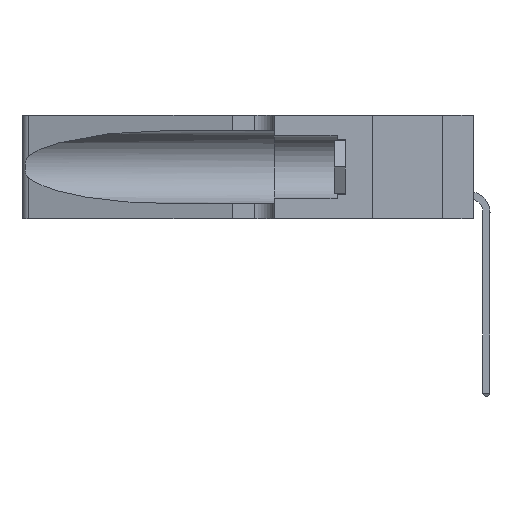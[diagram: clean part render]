
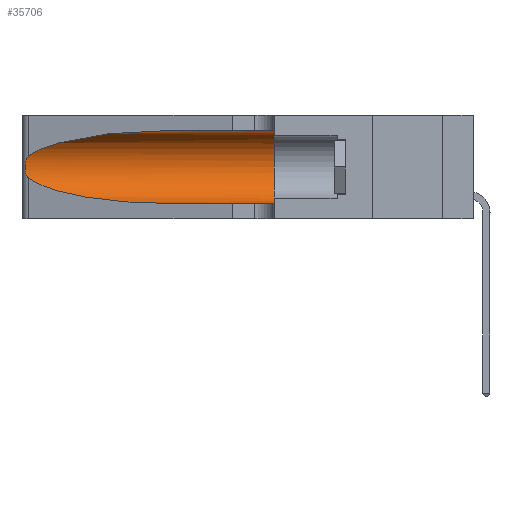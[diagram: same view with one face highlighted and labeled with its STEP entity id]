
A CAD part, left-side view. The second image highlights one B-rep face of the part: STEP entity #35706.
In plain terms, the highlighted cylindrical face has radius 3.308 mm (diameter 6.617 mm), a partial arc.
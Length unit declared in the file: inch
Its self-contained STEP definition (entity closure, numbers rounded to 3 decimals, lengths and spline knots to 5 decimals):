
#570 = CARTESIAN_POINT ( 'NONE',  ( 0.1305, 0.35, 0.05475 ) ) ;
#828 = EDGE_CURVE ( 'NONE', #36275, #28093, #7726, .T. ) ;
#1147 = CARTESIAN_POINT ( 'NONE',  ( 0.25487, 1.22718, 0.22369 ) ) ;
#1458 = CARTESIAN_POINT ( 'NONE',  ( 0.26075, 1.23896, 0.178 ) ) ;
#1589 = CARTESIAN_POINT ( 'NONE',  ( 0.25639, 1.23184, 0.21858 ) ) ;
#1686 = CARTESIAN_POINT ( 'NONE',  ( 0.1305, 0.72297, 0.31525 ) ) ;
#1888 = VERTEX_POINT ( 'NONE', #17448 ) ;
#1955 = CARTESIAN_POINT ( 'NONE',  ( 0.25487, 1.22718, 0.14631 ) ) ;
#2973 = DIRECTION ( 'NONE',  ( 0., -1., 0. ) ) ;
#3993 = CARTESIAN_POINT ( 'NONE',  ( 0.25555, 1.22994, 0.2215 ) ) ;
#4387 = CARTESIAN_POINT ( 'NONE',  ( 0.26017, 1.23833, 0.17102 ) ) ;
#5636 = EDGE_CURVE ( 'NONE', #1888, #11898, #5733, .T. ) ;
#5733 = CIRCLE ( 'NONE', #7338, 0.13025 ) ;
#6568 = CARTESIAN_POINT ( 'NONE',  ( 0.25487, 1.22718, 0.14631 ) ) ;
#7338 = AXIS2_PLACEMENT_3D ( 'NONE', #31438, #34355, #36896 ) ;
#7726 =( BOUNDED_CURVE ( )  B_SPLINE_CURVE ( 3, ( #1955, #13411, #25241, #36933 ),
 .UNSPECIFIED., .F., .T. ) 
 B_SPLINE_CURVE_WITH_KNOTS ( ( 4, 4 ),
 ( 3.44316, 4.71239 ),
 .UNSPECIFIED. ) 
 CURVE ( )  GEOMETRIC_REPRESENTATION_ITEM ( )  RATIONAL_B_SPLINE_CURVE ( ( 1., 0.87, 0.87, 1. ) ) 
 REPRESENTATION_ITEM ( '' )  );
#7829 = EDGE_LOOP ( 'NONE', ( #23922, #30203, #32178, #22317, #20930, #14837 ) ) ;
#7973 = CARTESIAN_POINT ( 'NONE',  ( 0.1305, 0.72297, 0.31525 ) ) ;
#8555 = VECTOR ( 'NONE', #23010, 39.37008 ) ;
#10827 = AXIS2_PLACEMENT_3D ( 'NONE', #21777, #24721, #27781 ) ;
#11898 = VERTEX_POINT ( 'NONE', #570 ) ;
#12617 = LINE ( 'NONE', #14281, #8555 ) ;
#13159 = CARTESIAN_POINT ( 'NONE',  ( 0.25639, 1.23186, 0.15144 ) ) ;
#13266 = CARTESIAN_POINT ( 'NONE',  ( 0.25487, 1.22718, 0.22369 ) ) ;
#13324 = EDGE_CURVE ( 'NONE', #18718, #1888, #12617, .T. ) ;
#13411 = CARTESIAN_POINT ( 'NONE',  ( 0.2373, 1.15595, 0.08982 ) ) ;
#14281 = CARTESIAN_POINT ( 'NONE',  ( 0.1305, 1.61858, 0.31525 ) ) ;
#14837 = ORIENTED_EDGE ( 'NONE', *, *, #13324, .F. ) ;
#16823 = EDGE_CURVE ( 'NONE', #18718, #19462, #18973, .T. ) ;
#17448 = CARTESIAN_POINT ( 'NONE',  ( 0.1305, 0.35, 0.31525 ) ) ;
#18718 = VERTEX_POINT ( 'NONE', #7973 ) ;
#18906 = CARTESIAN_POINT ( 'NONE',  ( 0.25487, 1.22718, 0.22369 ) ) ;
#18973 =( BOUNDED_CURVE ( )  B_SPLINE_CURVE ( 3, ( #1686, #36417, #36657, #13266 ),
 .UNSPECIFIED., .F., .T. ) 
 B_SPLINE_CURVE_WITH_KNOTS ( ( 4, 4 ),
 ( 1.5708, 2.84003 ),
 .UNSPECIFIED. ) 
 CURVE ( )  GEOMETRIC_REPRESENTATION_ITEM ( )  RATIONAL_B_SPLINE_CURVE ( ( 1., 0.87, 0.87, 1. ) ) 
 REPRESENTATION_ITEM ( '' )  );
#19462 = VERTEX_POINT ( 'NONE', #1147 ) ;
#20486 = EDGE_CURVE ( 'NONE', #28093, #11898, #28164, .T. ) ;
#20930 = ORIENTED_EDGE ( 'NONE', *, *, #5636, .F. ) ;
#21243 = B_SPLINE_CURVE_WITH_KNOTS ( 'NONE', 3,
 ( #18906, #3993, #1589, #36179, #30449, #24354, #30182, #1458, #4387, #33121, #24759, #13159, #22460, #27821 ),
 .UNSPECIFIED., .F., .F.,
 ( 4, 2, 2, 2, 2, 2, 4 ),
 ( 0., 0.00027, 0.00053, 0.00107, 0.0016, 0.00187, 0.00214 ),
 .UNSPECIFIED. ) ;
#21777 = CARTESIAN_POINT ( 'NONE',  ( 0.1305, 1.61858, 0.185 ) ) ;
#22317 = ORIENTED_EDGE ( 'NONE', *, *, #20486, .T. ) ;
#22460 = CARTESIAN_POINT ( 'NONE',  ( 0.25555, 1.22993, 0.14849 ) ) ;
#22715 = VECTOR ( 'NONE', #2973, 39.37008 ) ;
#23010 = DIRECTION ( 'NONE',  ( 0., -1., 0. ) ) ;
#23922 = ORIENTED_EDGE ( 'NONE', *, *, #16823, .T. ) ;
#24091 = EDGE_CURVE ( 'NONE', #19462, #36275, #21243, .T. ) ;
#24354 = CARTESIAN_POINT ( 'NONE',  ( 0.26018, 1.23835, 0.19895 ) ) ;
#24721 = DIRECTION ( 'NONE',  ( 0., -1., 0. ) ) ;
#24759 = CARTESIAN_POINT ( 'NONE',  ( 0.25789, 1.23486, 0.15765 ) ) ;
#25241 = CARTESIAN_POINT ( 'NONE',  ( 0.18966, 0.96281, 0.05475 ) ) ;
#25512 = FACE_OUTER_BOUND ( 'NONE', #7829, .T. ) ;
#27781 = DIRECTION ( 'NONE',  ( 0., 0., -1. ) ) ;
#27821 = CARTESIAN_POINT ( 'NONE',  ( 0.25487, 1.22718, 0.14631 ) ) ;
#28093 = VERTEX_POINT ( 'NONE', #28925 ) ;
#28164 = LINE ( 'NONE', #29056, #22715 ) ;
#28925 = CARTESIAN_POINT ( 'NONE',  ( 0.1305, 0.72297, 0.05475 ) ) ;
#29056 = CARTESIAN_POINT ( 'NONE',  ( 0.1305, 1.61858, 0.05475 ) ) ;
#30182 = CARTESIAN_POINT ( 'NONE',  ( 0.26075, 1.23896, 0.19203 ) ) ;
#30203 = ORIENTED_EDGE ( 'NONE', *, *, #24091, .T. ) ;
#30449 = CARTESIAN_POINT ( 'NONE',  ( 0.25854, 1.2359, 0.20912 ) ) ;
#31438 = CARTESIAN_POINT ( 'NONE',  ( 0.1305, 0.35, 0.185 ) ) ;
#32178 = ORIENTED_EDGE ( 'NONE', *, *, #828, .T. ) ;
#32282 = CYLINDRICAL_SURFACE ( 'NONE', #10827, 0.13025 ) ;
#33121 = CARTESIAN_POINT ( 'NONE',  ( 0.25856, 1.23593, 0.16098 ) ) ;
#34355 = DIRECTION ( 'NONE',  ( 0., 1., 0. ) ) ;
#35706 = ADVANCED_FACE ( 'NONE', ( #25512 ), #32282, .F. ) ;
#36179 = CARTESIAN_POINT ( 'NONE',  ( 0.25787, 1.23484, 0.2124 ) ) ;
#36275 = VERTEX_POINT ( 'NONE', #6568 ) ;
#36417 = CARTESIAN_POINT ( 'NONE',  ( 0.18966, 0.96281, 0.31525 ) ) ;
#36657 = CARTESIAN_POINT ( 'NONE',  ( 0.2373, 1.15595, 0.28018 ) ) ;
#36896 = DIRECTION ( 'NONE',  ( 0., 0., 1. ) ) ;
#36933 = CARTESIAN_POINT ( 'NONE',  ( 0.1305, 0.72297, 0.05475 ) ) ;
